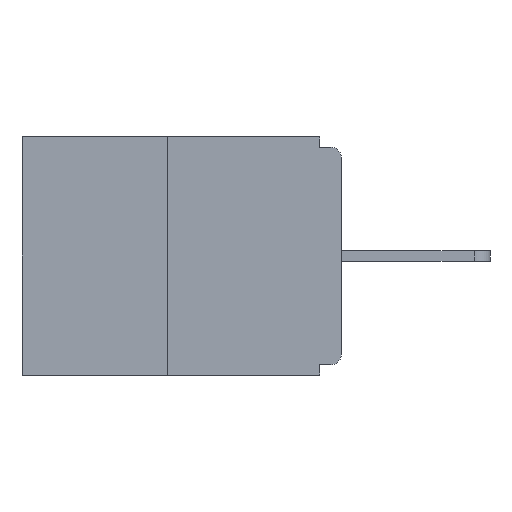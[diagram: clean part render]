
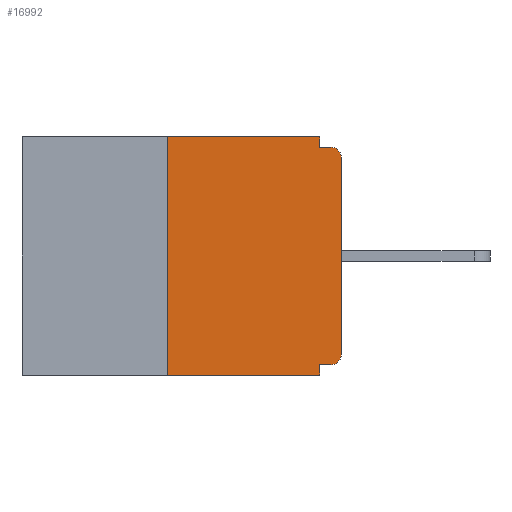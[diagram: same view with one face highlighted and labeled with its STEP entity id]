
A CAD part, left-side view. The second image highlights one B-rep face of the part: STEP entity #16992.
In plain terms, the highlighted planar face has unit normal (-1, 0, 0).
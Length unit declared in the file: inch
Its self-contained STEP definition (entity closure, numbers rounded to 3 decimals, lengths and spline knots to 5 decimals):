
#33 = DIRECTION ( 'NONE',  ( 0., -1., 0. ) ) ;
#335 = CARTESIAN_POINT ( 'NONE',  ( 0., 0.015, -0.015 ) ) ;
#394 = DIRECTION ( 'NONE',  ( -1., 0., 0. ) ) ;
#598 = CIRCLE ( 'NONE', #12284, 0.015 ) ;
#879 = ORIENTED_EDGE ( 'NONE', *, *, #5938, .T. ) ;
#1219 = LINE ( 'NONE', #13626, #17964 ) ;
#1307 = EDGE_CURVE ( 'NONE', #11649, #8303, #15609, .T. ) ;
#1611 = CARTESIAN_POINT ( 'NONE',  ( 0., 0.031, -0.343 ) ) ;
#1760 = VECTOR ( 'NONE', #33, 39.37008 ) ;
#1974 = DIRECTION ( 'NONE',  ( 0., 1., 0. ) ) ;
#2582 = DIRECTION ( 'NONE',  ( 0., 0., 1. ) ) ;
#2625 = VECTOR ( 'NONE', #19924, 39.37008 ) ;
#2667 = DIRECTION ( 'NONE',  ( 0., 0., -1. ) ) ;
#2699 = DIRECTION ( 'NONE',  ( 1., 0., 0. ) ) ;
#2911 = ORIENTED_EDGE ( 'NONE', *, *, #5202, .F. ) ;
#3318 = LINE ( 'NONE', #11828, #12040 ) ;
#3607 = EDGE_CURVE ( 'NONE', #16854, #16769, #6200, .T. ) ;
#3875 = CIRCLE ( 'NONE', #13151, 0.015 ) ;
#3965 = CARTESIAN_POINT ( 'NONE',  ( 0., 0.031, -0.343 ) ) ;
#4026 = ORIENTED_EDGE ( 'NONE', *, *, #19612, .T. ) ;
#4112 = EDGE_CURVE ( 'NONE', #16769, #10699, #8995, .T. ) ;
#4191 = VERTEX_POINT ( 'NONE', #6182 ) ;
#4618 = VECTOR ( 'NONE', #2667, 39.37008 ) ;
#5005 = CARTESIAN_POINT ( 'NONE',  ( 0., 0.015, -0.328 ) ) ;
#5202 = EDGE_CURVE ( 'NONE', #10699, #20905, #19671, .T. ) ;
#5652 = ORIENTED_EDGE ( 'NONE', *, *, #3607, .F. ) ;
#5938 = EDGE_CURVE ( 'NONE', #9561, #20034, #598, .T. ) ;
#6182 = CARTESIAN_POINT ( 'NONE',  ( 0., 0.25, -0.343 ) ) ;
#6200 = LINE ( 'NONE', #12274, #1760 ) ;
#6837 = CARTESIAN_POINT ( 'NONE',  ( 0., 0.031, 0. ) ) ;
#6924 = CARTESIAN_POINT ( 'NONE',  ( 0., 0.015, -0.313 ) ) ;
#6951 = AXIS2_PLACEMENT_3D ( 'NONE', #17226, #2699, #14099 ) ;
#7332 = FACE_OUTER_BOUND ( 'NONE', #8429, .T. ) ;
#8303 = VERTEX_POINT ( 'NONE', #1611 ) ;
#8363 = LINE ( 'NONE', #10056, #12159 ) ;
#8429 = EDGE_LOOP ( 'NONE', ( #5652, #8494, #4026, #11345, #10081, #879, #11645, #20484, #2911, #17107 ) ) ;
#8494 = ORIENTED_EDGE ( 'NONE', *, *, #14048, .F. ) ;
#8570 = DIRECTION ( 'NONE',  ( 0., 0., -1. ) ) ;
#8995 = LINE ( 'NONE', #6837, #4618 ) ;
#9561 = VERTEX_POINT ( 'NONE', #5005 ) ;
#10056 = CARTESIAN_POINT ( 'NONE',  ( 0., 0.46, -0.343 ) ) ;
#10081 = ORIENTED_EDGE ( 'NONE', *, *, #13713, .F. ) ;
#10345 = CARTESIAN_POINT ( 'NONE',  ( 0., 0.015, -0.03 ) ) ;
#10699 = VERTEX_POINT ( 'NONE', #20891 ) ;
#10825 = CARTESIAN_POINT ( 'NONE',  ( 0., 0.25, 0. ) ) ;
#11345 = ORIENTED_EDGE ( 'NONE', *, *, #1307, .F. ) ;
#11645 = ORIENTED_EDGE ( 'NONE', *, *, #13812, .T. ) ;
#11649 = VERTEX_POINT ( 'NONE', #15735 ) ;
#11828 = CARTESIAN_POINT ( 'NONE',  ( 0., 0., -0.328 ) ) ;
#11939 = DIRECTION ( 'NONE',  ( 0., 0., -1. ) ) ;
#12040 = VECTOR ( 'NONE', #1974, 39.37008 ) ;
#12159 = VECTOR ( 'NONE', #17940, 39.37008 ) ;
#12274 = CARTESIAN_POINT ( 'NONE',  ( 0., 0.46, 0. ) ) ;
#12284 = AXIS2_PLACEMENT_3D ( 'NONE', #6924, #18118, #8570 ) ;
#12508 = PLANE ( 'NONE',  #6951 ) ;
#12655 = EDGE_CURVE ( 'NONE', #19187, #20905, #3875, .T. ) ;
#12740 = CARTESIAN_POINT ( 'NONE',  ( 0., 0., -0.313 ) ) ;
#13151 = AXIS2_PLACEMENT_3D ( 'NONE', #10345, #394, #11939 ) ;
#13240 = CARTESIAN_POINT ( 'NONE',  ( 0., 0., -0.03 ) ) ;
#13492 = CARTESIAN_POINT ( 'NONE',  ( 0., 0.031, 0. ) ) ;
#13516 = VECTOR ( 'NONE', #2582, 39.37008 ) ;
#13626 = CARTESIAN_POINT ( 'NONE',  ( 0., 0., 0. ) ) ;
#13713 = EDGE_CURVE ( 'NONE', #9561, #11649, #3318, .T. ) ;
#13761 = CARTESIAN_POINT ( 'NONE',  ( 0., 0.25, 0. ) ) ;
#13812 = EDGE_CURVE ( 'NONE', #20034, #19187, #1219, .T. ) ;
#14048 = EDGE_CURVE ( 'NONE', #4191, #16854, #17720, .T. ) ;
#14099 = DIRECTION ( 'NONE',  ( 0., 0., -1. ) ) ;
#14956 = VECTOR ( 'NONE', #19550, 39.37008 ) ;
#15609 = LINE ( 'NONE', #3965, #2625 ) ;
#15735 = CARTESIAN_POINT ( 'NONE',  ( 0., 0.031, -0.328 ) ) ;
#16769 = VERTEX_POINT ( 'NONE', #13492 ) ;
#16822 = DIRECTION ( 'NONE',  ( 0., 0., 1. ) ) ;
#16854 = VERTEX_POINT ( 'NONE', #13761 ) ;
#16992 = ADVANCED_FACE ( 'NONE', ( #7332 ), #12508, .F. ) ;
#17107 = ORIENTED_EDGE ( 'NONE', *, *, #4112, .F. ) ;
#17226 = CARTESIAN_POINT ( 'NONE',  ( 0., 0.46, 0. ) ) ;
#17720 = LINE ( 'NONE', #10825, #13516 ) ;
#17940 = DIRECTION ( 'NONE',  ( 0., -1., 0. ) ) ;
#17964 = VECTOR ( 'NONE', #16822, 39.37008 ) ;
#18118 = DIRECTION ( 'NONE',  ( -1., 0., 0. ) ) ;
#19187 = VERTEX_POINT ( 'NONE', #13240 ) ;
#19434 = CARTESIAN_POINT ( 'NONE',  ( 0., 0., -0.015 ) ) ;
#19550 = DIRECTION ( 'NONE',  ( 0., -1., 0. ) ) ;
#19612 = EDGE_CURVE ( 'NONE', #4191, #8303, #8363, .T. ) ;
#19671 = LINE ( 'NONE', #19434, #14956 ) ;
#19924 = DIRECTION ( 'NONE',  ( 0., 0., -1. ) ) ;
#20034 = VERTEX_POINT ( 'NONE', #12740 ) ;
#20484 = ORIENTED_EDGE ( 'NONE', *, *, #12655, .T. ) ;
#20891 = CARTESIAN_POINT ( 'NONE',  ( 0., 0.031, -0.015 ) ) ;
#20905 = VERTEX_POINT ( 'NONE', #335 ) ;
